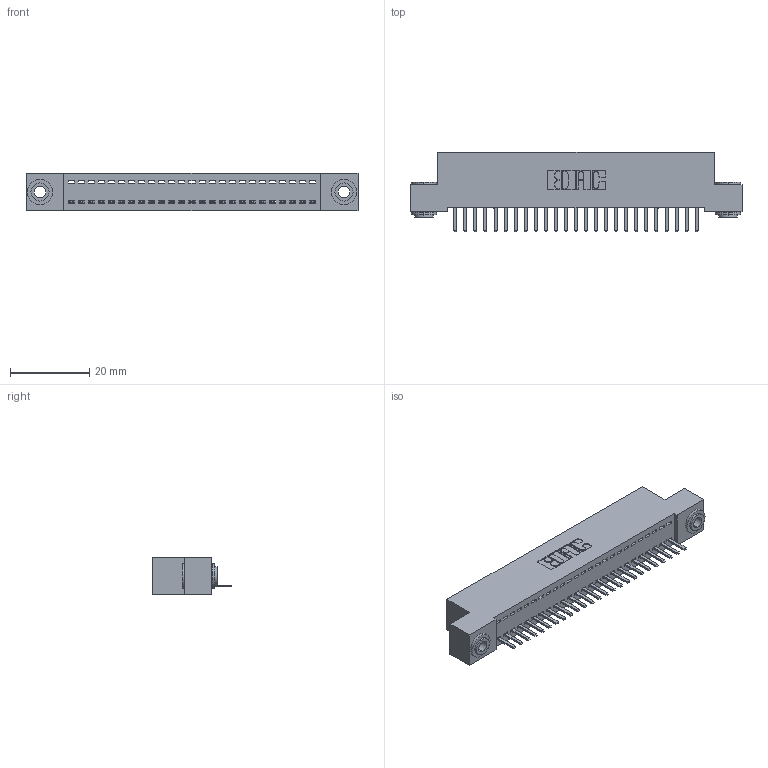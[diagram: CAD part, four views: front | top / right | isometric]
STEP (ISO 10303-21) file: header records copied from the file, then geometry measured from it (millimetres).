
FILE_DESCRIPTION (( 'STEP AP203' ), '1' );
FILE_NAME ('342-025-520-103.STEP', '2019-10-02T00:26:40', ( '' ), ( '' ), 'SwSTEP 2.0', 'SolidWorks 2016', '' );
FILE_SCHEMA (( 'CONFIG_CONTROL_DESIGN' ));
Length unit declared in the file: inch
Products named in the file (4): 342 Part_.156 TH; 345-292-001_345-293-120; 342-250-002_345-250-002-102; 342-025-520-103
Assembly tree (28 placements, depth 2):
  342-025-520-103
    342 Part_.156 TH
    345-292-001_345-293-120  x25
    342-250-002_345-250-002-102  x2
Bounding box: 83.82 x 20.02 x 9.4 mm (x, y, z)
Volume: 7237.6 mm3; surface area: 10306.9 mm2
Topology: 28 solids, 28 shells, 1698 faces, 4975 edges, 3246 vertices
Faces by surface type: plane 1176, cylinder 514, cone 8
Entity records: 18114 total; most frequent: CARTESIAN_POINT 3116, ORIENTED_EDGE 3058, DIRECTION 2685, EDGE_CURVE 1529, LINE 1373, VECTOR 1373, VERTEX_POINT 1014, AXIS2_PLACEMENT_3D 656
